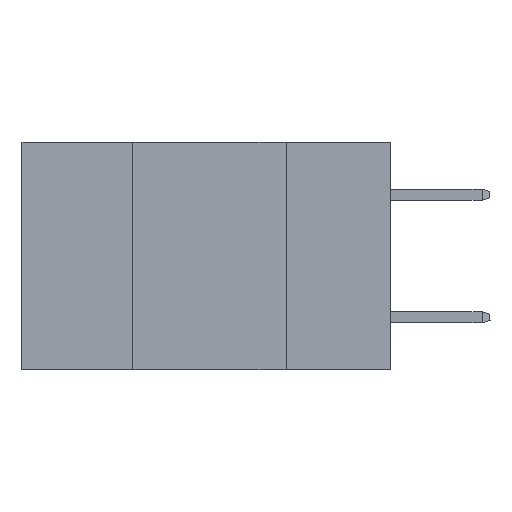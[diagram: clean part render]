
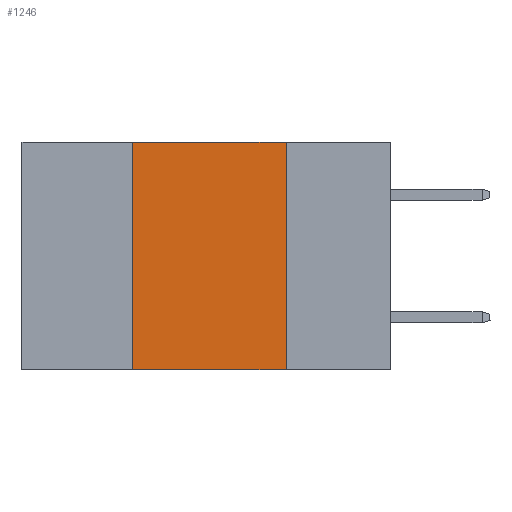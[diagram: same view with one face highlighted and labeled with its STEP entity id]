
A CAD part, left-side view. The second image highlights one B-rep face of the part: STEP entity #1246.
In plain terms, the highlighted planar face has unit normal (-1, 0, 0).
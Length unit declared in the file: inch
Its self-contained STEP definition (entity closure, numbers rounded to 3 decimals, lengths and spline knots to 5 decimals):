
#591 = CARTESIAN_POINT ( 'NONE',  ( 0., 0.42, 0. ) ) ;
#1079 = EDGE_CURVE ( 'NONE', #11809, #5594, #2544, .T. ) ;
#1219 = EDGE_CURVE ( 'NONE', #5594, #15915, #13456, .T. ) ;
#1246 = ADVANCED_FACE ( 'NONE', ( #17124 ), #2086, .F. ) ;
#2086 = PLANE ( 'NONE',  #10618 ) ;
#2544 = LINE ( 'NONE', #591, #6798 ) ;
#2831 = VECTOR ( 'NONE', #19862, 39.37008 ) ;
#3081 = CARTESIAN_POINT ( 'NONE',  ( 0., 0.17, 0. ) ) ;
#4948 = LINE ( 'NONE', #3081, #8419 ) ;
#5373 = DIRECTION ( 'NONE',  ( 0., 0., 1. ) ) ;
#5594 = VERTEX_POINT ( 'NONE', #22456 ) ;
#6113 = VERTEX_POINT ( 'NONE', #13081 ) ;
#6798 = VECTOR ( 'NONE', #5373, 39.37008 ) ;
#6961 = DIRECTION ( 'NONE',  ( 1., 0., 0. ) ) ;
#7709 = CARTESIAN_POINT ( 'NONE',  ( 0., 0.17, 0. ) ) ;
#8419 = VECTOR ( 'NONE', #17407, 39.37008 ) ;
#8770 = VECTOR ( 'NONE', #14486, 39.37008 ) ;
#10056 = ORIENTED_EDGE ( 'NONE', *, *, #1079, .F. ) ;
#10618 = AXIS2_PLACEMENT_3D ( 'NONE', #11407, #6961, #22987 ) ;
#11407 = CARTESIAN_POINT ( 'NONE',  ( 0., 0.6, 0. ) ) ;
#11809 = VERTEX_POINT ( 'NONE', #14952 ) ;
#11895 = ORIENTED_EDGE ( 'NONE', *, *, #18368, .F. ) ;
#13081 = CARTESIAN_POINT ( 'NONE',  ( 0., 0.17, -0.37 ) ) ;
#13456 = LINE ( 'NONE', #20698, #8770 ) ;
#14486 = DIRECTION ( 'NONE',  ( 0., -1., 0. ) ) ;
#14952 = CARTESIAN_POINT ( 'NONE',  ( 0., 0.42, -0.37 ) ) ;
#15915 = VERTEX_POINT ( 'NONE', #7709 ) ;
#16265 = CARTESIAN_POINT ( 'NONE',  ( 0., 0.6, -0.37 ) ) ;
#16395 = ORIENTED_EDGE ( 'NONE', *, *, #1219, .F. ) ;
#17119 = LINE ( 'NONE', #16265, #2831 ) ;
#17124 = FACE_OUTER_BOUND ( 'NONE', #18744, .T. ) ;
#17407 = DIRECTION ( 'NONE',  ( 0., 0., -1. ) ) ;
#17798 = ORIENTED_EDGE ( 'NONE', *, *, #23185, .T. ) ;
#18368 = EDGE_CURVE ( 'NONE', #15915, #6113, #4948, .T. ) ;
#18744 = EDGE_LOOP ( 'NONE', ( #11895, #16395, #10056, #17798 ) ) ;
#19862 = DIRECTION ( 'NONE',  ( 0., -1., 0. ) ) ;
#20698 = CARTESIAN_POINT ( 'NONE',  ( 0., 0.6, 0. ) ) ;
#22456 = CARTESIAN_POINT ( 'NONE',  ( 0., 0.42, 0. ) ) ;
#22987 = DIRECTION ( 'NONE',  ( 0., 0., -1. ) ) ;
#23185 = EDGE_CURVE ( 'NONE', #11809, #6113, #17119, .T. ) ;
